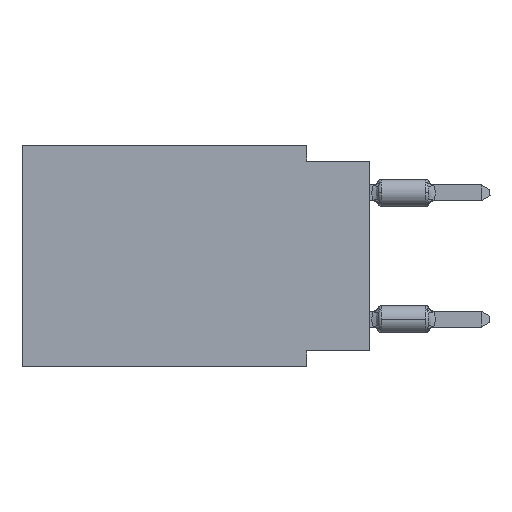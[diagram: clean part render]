
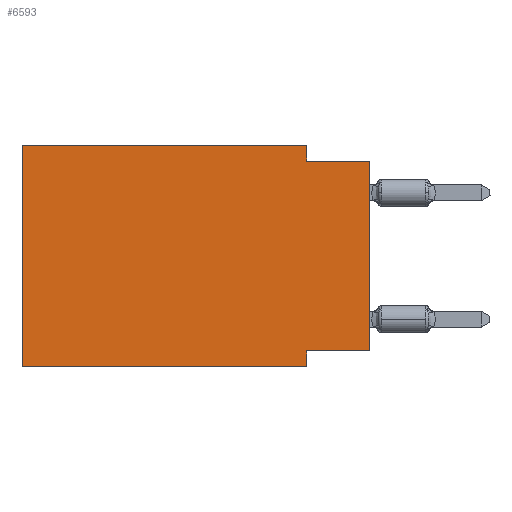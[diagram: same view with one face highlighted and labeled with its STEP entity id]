
A CAD part, left-side view. The second image highlights one B-rep face of the part: STEP entity #6593.
In plain terms, the highlighted planar face has unit normal (-1, 0, 0).
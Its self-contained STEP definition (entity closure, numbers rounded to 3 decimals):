
#120 = CARTESIAN_POINT ( 'NONE',  ( 0., 0., -0.635 ) ) ;
#190 = ORIENTED_EDGE ( 'NONE', *, *, #32295, .T. ) ;
#417 = VECTOR ( 'NONE', #5462, 1000. ) ;
#620 = VECTOR ( 'NONE', #48572, 1000. ) ;
#743 = ORIENTED_EDGE ( 'NONE', *, *, #45646, .F. ) ;
#2133 = VECTOR ( 'NONE', #42346, 1000. ) ;
#2275 = VERTEX_POINT ( 'NONE', #30227 ) ;
#2354 = CARTESIAN_POINT ( 'NONE',  ( 0., 2.54, -8.89 ) ) ;
#2662 = CARTESIAN_POINT ( 'NONE',  ( 0., 2.54, 0. ) ) ;
#3812 = EDGE_CURVE ( 'NONE', #44488, #33560, #41834, .T. ) ;
#5218 = LINE ( 'NONE', #47143, #12188 ) ;
#5462 = DIRECTION ( 'NONE',  ( 0., 0., 1. ) ) ;
#6184 = ORIENTED_EDGE ( 'NONE', *, *, #11324, .F. ) ;
#6593 = ADVANCED_FACE ( 'NONE', ( #48522 ), #25477, .F. ) ;
#6635 = CARTESIAN_POINT ( 'NONE',  ( 0., 13.97, 0. ) ) ;
#7943 = CARTESIAN_POINT ( 'NONE',  ( 0., 2.54, -8.89 ) ) ;
#8064 = ORIENTED_EDGE ( 'NONE', *, *, #29008, .F. ) ;
#8699 = DIRECTION ( 'NONE',  ( 0., 0., -1. ) ) ;
#9699 = VECTOR ( 'NONE', #17489, 1000. ) ;
#10385 = CARTESIAN_POINT ( 'NONE',  ( 0., 0., -8.255 ) ) ;
#10827 = ORIENTED_EDGE ( 'NONE', *, *, #3812, .F. ) ;
#10965 = AXIS2_PLACEMENT_3D ( 'NONE', #6635, #25976, #32905 ) ;
#11324 = EDGE_CURVE ( 'NONE', #44986, #2275, #14203, .T. ) ;
#11825 = LINE ( 'NONE', #15317, #2133 ) ;
#12188 = VECTOR ( 'NONE', #8699, 1000. ) ;
#13164 = EDGE_CURVE ( 'NONE', #33560, #31831, #18227, .T. ) ;
#13217 = VECTOR ( 'NONE', #19149, 1000. ) ;
#13534 = VECTOR ( 'NONE', #19541, 1000. ) ;
#14203 = LINE ( 'NONE', #21382, #39796 ) ;
#15117 = EDGE_CURVE ( 'NONE', #44488, #22853, #27555, .T. ) ;
#15200 = LINE ( 'NONE', #30320, #13217 ) ;
#15317 = CARTESIAN_POINT ( 'NONE',  ( 0., 13.97, 0. ) ) ;
#16398 = CARTESIAN_POINT ( 'NONE',  ( 0., 0., 0. ) ) ;
#17021 = VERTEX_POINT ( 'NONE', #18055 ) ;
#17489 = DIRECTION ( 'NONE',  ( 0., 0., -1. ) ) ;
#18055 = CARTESIAN_POINT ( 'NONE',  ( 0., 2.54, -0.635 ) ) ;
#18227 = LINE ( 'NONE', #2354, #9699 ) ;
#19149 = DIRECTION ( 'NONE',  ( 0., -1., 0. ) ) ;
#19541 = DIRECTION ( 'NONE',  ( 0., -1., 0. ) ) ;
#20956 = ORIENTED_EDGE ( 'NONE', *, *, #35889, .F. ) ;
#21382 = CARTESIAN_POINT ( 'NONE',  ( 0., 13.97, 0. ) ) ;
#22853 = VERTEX_POINT ( 'NONE', #120 ) ;
#25477 = PLANE ( 'NONE',  #10965 ) ;
#25976 = DIRECTION ( 'NONE',  ( 1., 0., 0. ) ) ;
#26254 = CARTESIAN_POINT ( 'NONE',  ( 0., 13.97, -8.89 ) ) ;
#27555 = LINE ( 'NONE', #16398, #417 ) ;
#29008 = EDGE_CURVE ( 'NONE', #17021, #22853, #15200, .T. ) ;
#29303 = DIRECTION ( 'NONE',  ( 0., 0., 1. ) ) ;
#30227 = CARTESIAN_POINT ( 'NONE',  ( 0., 13.97, 0. ) ) ;
#30320 = CARTESIAN_POINT ( 'NONE',  ( 0., 0., -0.635 ) ) ;
#30606 = CARTESIAN_POINT ( 'NONE',  ( 0., 0., -8.255 ) ) ;
#31831 = VERTEX_POINT ( 'NONE', #7943 ) ;
#32295 = EDGE_CURVE ( 'NONE', #44986, #31831, #45345, .T. ) ;
#32905 = DIRECTION ( 'NONE',  ( 0., 0., -1. ) ) ;
#33560 = VERTEX_POINT ( 'NONE', #44330 ) ;
#35889 = EDGE_CURVE ( 'NONE', #48776, #17021, #5218, .T. ) ;
#35966 = CARTESIAN_POINT ( 'NONE',  ( 0., 13.97, -8.89 ) ) ;
#36475 = ORIENTED_EDGE ( 'NONE', *, *, #13164, .F. ) ;
#39796 = VECTOR ( 'NONE', #29303, 1000. ) ;
#41834 = LINE ( 'NONE', #10385, #620 ) ;
#42346 = DIRECTION ( 'NONE',  ( 0., -1., 0. ) ) ;
#44330 = CARTESIAN_POINT ( 'NONE',  ( 0., 2.54, -8.255 ) ) ;
#44488 = VERTEX_POINT ( 'NONE', #30606 ) ;
#44986 = VERTEX_POINT ( 'NONE', #35966 ) ;
#45345 = LINE ( 'NONE', #26254, #13534 ) ;
#45418 = ORIENTED_EDGE ( 'NONE', *, *, #15117, .T. ) ;
#45646 = EDGE_CURVE ( 'NONE', #2275, #48776, #11825, .T. ) ;
#46790 = EDGE_LOOP ( 'NONE', ( #45418, #8064, #20956, #743, #6184, #190, #36475, #10827 ) ) ;
#47143 = CARTESIAN_POINT ( 'NONE',  ( 0., 2.54, 0. ) ) ;
#48522 = FACE_OUTER_BOUND ( 'NONE', #46790, .T. ) ;
#48572 = DIRECTION ( 'NONE',  ( 0., 1., 0. ) ) ;
#48776 = VERTEX_POINT ( 'NONE', #2662 ) ;
